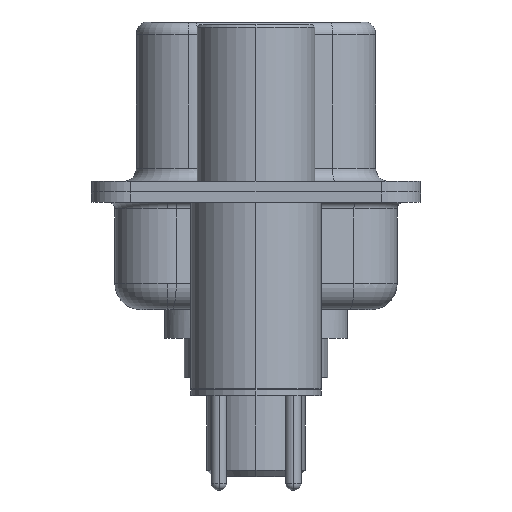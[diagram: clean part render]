
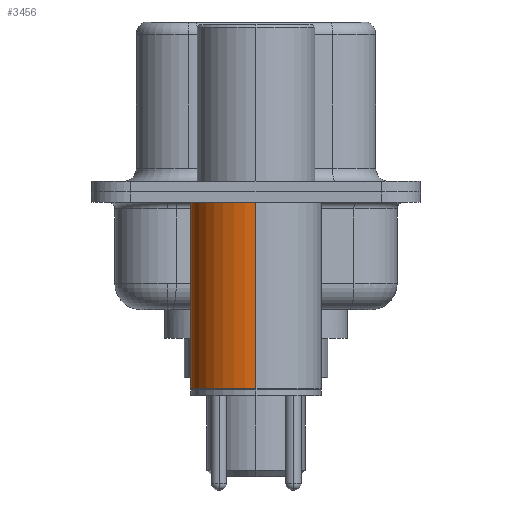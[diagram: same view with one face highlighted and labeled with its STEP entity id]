
A CAD part, left-side view. The second image highlights one B-rep face of the part: STEP entity #3456.
In plain terms, the highlighted cylindrical face has radius 2.5 mm (diameter 5 mm), a partial arc.
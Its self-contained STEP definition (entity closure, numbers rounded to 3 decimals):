
#48 = DIRECTION ( 'NONE',  ( 1., 0., 0. ) ) ;
#511 = EDGE_CURVE ( 'NONE', #13942, #15883, #12248, .T. ) ;
#1018 = EDGE_CURVE ( 'NONE', #13359, #2414, #2859, .T. ) ;
#1257 = EDGE_CURVE ( 'NONE', #2414, #15883, #12047, .T. ) ;
#1324 = AXIS2_PLACEMENT_3D ( 'NONE', #14265, #6974, #15476 ) ;
#1331 = CARTESIAN_POINT ( 'NONE',  ( 0., 0., 0.581 ) ) ;
#2099 = EDGE_LOOP ( 'NONE', ( #3101, #4648, #7723, #7146 ) ) ;
#2414 = VERTEX_POINT ( 'NONE', #15312 ) ;
#2859 = LINE ( 'NONE', #4931, #9015 ) ;
#3101 = ORIENTED_EDGE ( 'NONE', *, *, #13340, .T. ) ;
#3225 = DIRECTION ( 'NONE',  ( 0., 0., 1. ) ) ;
#3456 = ADVANCED_FACE ( 'NONE', ( #6794 ), #3896, .T. ) ;
#3896 = CYLINDRICAL_SURFACE ( 'NONE', #5848, 2.5 ) ;
#4648 = ORIENTED_EDGE ( 'NONE', *, *, #511, .T. ) ;
#4886 = DIRECTION ( 'NONE',  ( 1., 0., 0. ) ) ;
#4931 = CARTESIAN_POINT ( 'NONE',  ( 2.5, 0., 0.581 ) ) ;
#5449 = CARTESIAN_POINT ( 'NONE',  ( 0., 0., -0.4 ) ) ;
#5848 = AXIS2_PLACEMENT_3D ( 'NONE', #1331, #8581, #4886 ) ;
#6794 = FACE_OUTER_BOUND ( 'NONE', #2099, .T. ) ;
#6974 = DIRECTION ( 'NONE',  ( 0., 0., 1. ) ) ;
#7146 = ORIENTED_EDGE ( 'NONE', *, *, #1018, .F. ) ;
#7723 = ORIENTED_EDGE ( 'NONE', *, *, #1257, .F. ) ;
#7950 = CARTESIAN_POINT ( 'NONE',  ( -2.5, 0., -7.525 ) ) ;
#8581 = DIRECTION ( 'NONE',  ( 0., 0., 1. ) ) ;
#9015 = VECTOR ( 'NONE', #3225, 1000. ) ;
#9024 = VECTOR ( 'NONE', #11165, 1000. ) ;
#10379 = CARTESIAN_POINT ( 'NONE',  ( -2.5, 0., -0.4 ) ) ;
#11165 = DIRECTION ( 'NONE',  ( 0., 0., 1. ) ) ;
#11704 = CARTESIAN_POINT ( 'NONE',  ( -2.5, 0., 0.581 ) ) ;
#11913 = AXIS2_PLACEMENT_3D ( 'NONE', #5449, #14630, #48 ) ;
#12047 = CIRCLE ( 'NONE', #11913, 2.5 ) ;
#12248 = LINE ( 'NONE', #11704, #9024 ) ;
#13066 = CARTESIAN_POINT ( 'NONE',  ( 2.5, 0., -7.525 ) ) ;
#13340 = EDGE_CURVE ( 'NONE', #13359, #13942, #14387, .T. ) ;
#13359 = VERTEX_POINT ( 'NONE', #13066 ) ;
#13942 = VERTEX_POINT ( 'NONE', #7950 ) ;
#14265 = CARTESIAN_POINT ( 'NONE',  ( 0., 0., -7.525 ) ) ;
#14387 = CIRCLE ( 'NONE', #1324, 2.5 ) ;
#14630 = DIRECTION ( 'NONE',  ( 0., 0., 1. ) ) ;
#15312 = CARTESIAN_POINT ( 'NONE',  ( 2.5, 0., -0.4 ) ) ;
#15476 = DIRECTION ( 'NONE',  ( 1., 0., 0. ) ) ;
#15883 = VERTEX_POINT ( 'NONE', #10379 ) ;
